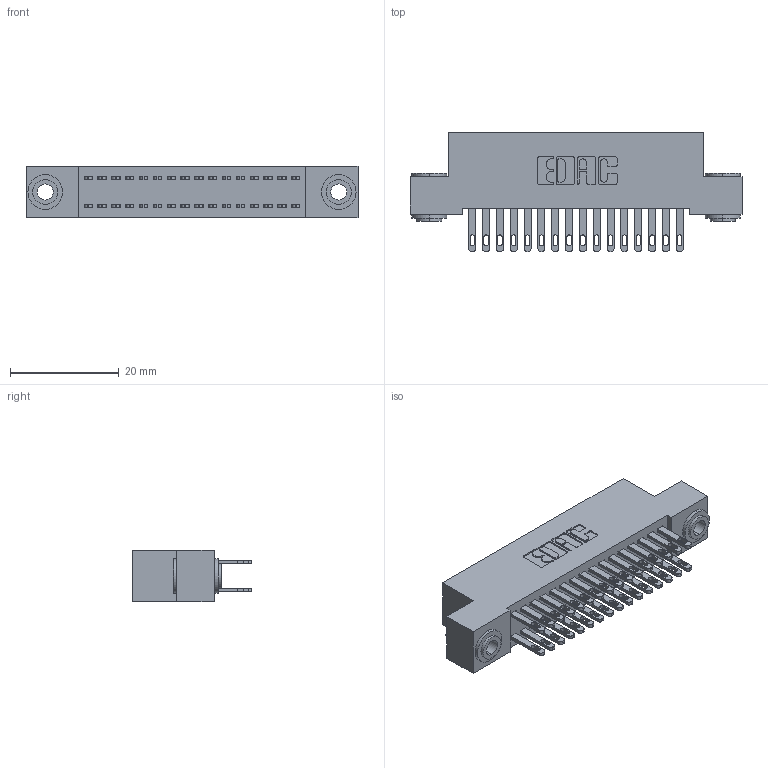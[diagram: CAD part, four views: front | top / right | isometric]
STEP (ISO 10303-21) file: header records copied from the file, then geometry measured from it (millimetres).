
FILE_DESCRIPTION (( 'STEP AP203' ), '1' );
FILE_NAME ('892-032-500-203.STEP', '2020-09-21T15:25:21', ( '' ), ( '' ), 'SwSTEP 2.0', 'SolidWorks 2020', '' );
FILE_SCHEMA (( 'CONFIG_CONTROL_DESIGN' ));
Length unit declared in the file: inch
Products named in the file (4): 342-250-002_345-250-002-102; 345-292-001_345-293-100; 842 Part_.156 TH; 892-032-500-203
Assembly tree (35 placements, depth 2):
  892-032-500-203
    842 Part_.156 TH
    345-292-001_345-293-100  x32
    342-250-002_345-250-002-102  x2
Bounding box: 60.96 x 21.85 x 9.4 mm (x, y, z)
Volume: 5474.8 mm3; surface area: 8791.4 mm2
Topology: 35 solids, 35 shells, 1684 faces, 5079 edges, 3382 vertices
Faces by surface type: plane 1036, cylinder 640, cone 8
Entity records: 14104 total; most frequent: CARTESIAN_POINT 2341, ORIENTED_EDGE 2270, DIRECTION 2081, EDGE_CURVE 1135, VECTOR 979, LINE 979, VERTEX_POINT 754, AXIS2_PLACEMENT_3D 551
